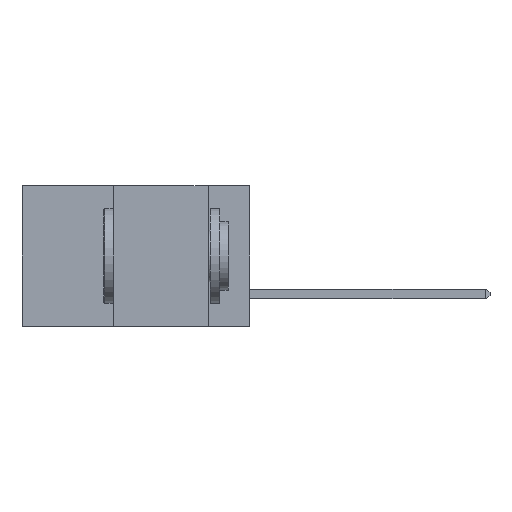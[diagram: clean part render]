
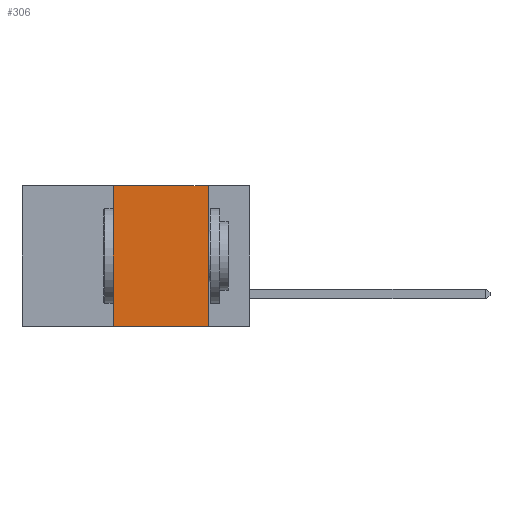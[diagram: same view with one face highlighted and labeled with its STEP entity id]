
A CAD part, left-side view. The second image highlights one B-rep face of the part: STEP entity #306.
In plain terms, the highlighted planar face has unit normal (-1, 0, 0).
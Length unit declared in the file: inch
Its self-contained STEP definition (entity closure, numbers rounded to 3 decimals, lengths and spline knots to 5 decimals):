
#206 = VERTEX_POINT ( 'NONE', #8502 ) ;
#213 = VECTOR ( 'NONE', #7571, 39.37008 ) ;
#306 = ADVANCED_FACE ( 'NONE', ( #6769 ), #4083, .F. ) ;
#423 = VERTEX_POINT ( 'NONE', #5645 ) ;
#651 = CARTESIAN_POINT ( 'NONE',  ( 0., 0.6, -0.37 ) ) ;
#3104 = EDGE_CURVE ( 'NONE', #423, #4857, #8348, .T. ) ;
#3624 = ORIENTED_EDGE ( 'NONE', *, *, #10114, .F. ) ;
#3804 = DIRECTION ( 'NONE',  ( 0., -1., 0. ) ) ;
#4070 = DIRECTION ( 'NONE',  ( 0., 0., -1. ) ) ;
#4083 = PLANE ( 'NONE',  #9086 ) ;
#4492 = VECTOR ( 'NONE', #3804, 39.37008 ) ;
#4645 = CARTESIAN_POINT ( 'NONE',  ( 0., 0.36, 0. ) ) ;
#4857 = VERTEX_POINT ( 'NONE', #4645 ) ;
#5047 = DIRECTION ( 'NONE',  ( 1., 0., 0. ) ) ;
#5493 = CARTESIAN_POINT ( 'NONE',  ( 0., 0.11, 0. ) ) ;
#5645 = CARTESIAN_POINT ( 'NONE',  ( 0., 0.36, -0.37 ) ) ;
#6074 = EDGE_CURVE ( 'NONE', #9720, #206, #8762, .T. ) ;
#6132 = DIRECTION ( 'NONE',  ( 0., -1., 0. ) ) ;
#6267 = EDGE_LOOP ( 'NONE', ( #9219, #3624, #9634, #8008 ) ) ;
#6391 = VECTOR ( 'NONE', #9741, 39.37008 ) ;
#6769 = FACE_OUTER_BOUND ( 'NONE', #6267, .T. ) ;
#6978 = LINE ( 'NONE', #9757, #8715 ) ;
#7297 = CARTESIAN_POINT ( 'NONE',  ( 0., 0.6, 0. ) ) ;
#7417 = CARTESIAN_POINT ( 'NONE',  ( 0., 0.11, 0. ) ) ;
#7571 = DIRECTION ( 'NONE',  ( 0., 0., -1. ) ) ;
#7779 = EDGE_CURVE ( 'NONE', #423, #206, #8190, .T. ) ;
#8008 = ORIENTED_EDGE ( 'NONE', *, *, #7779, .T. ) ;
#8190 = LINE ( 'NONE', #651, #4492 ) ;
#8348 = LINE ( 'NONE', #10040, #6391 ) ;
#8502 = CARTESIAN_POINT ( 'NONE',  ( 0., 0.11, -0.37 ) ) ;
#8715 = VECTOR ( 'NONE', #6132, 39.37008 ) ;
#8762 = LINE ( 'NONE', #7417, #213 ) ;
#9086 = AXIS2_PLACEMENT_3D ( 'NONE', #7297, #5047, #4070 ) ;
#9219 = ORIENTED_EDGE ( 'NONE', *, *, #6074, .F. ) ;
#9634 = ORIENTED_EDGE ( 'NONE', *, *, #3104, .F. ) ;
#9720 = VERTEX_POINT ( 'NONE', #5493 ) ;
#9741 = DIRECTION ( 'NONE',  ( 0., 0., 1. ) ) ;
#9757 = CARTESIAN_POINT ( 'NONE',  ( 0., 0.6, 0. ) ) ;
#10040 = CARTESIAN_POINT ( 'NONE',  ( 0., 0.36, 0. ) ) ;
#10114 = EDGE_CURVE ( 'NONE', #4857, #9720, #6978, .T. ) ;
